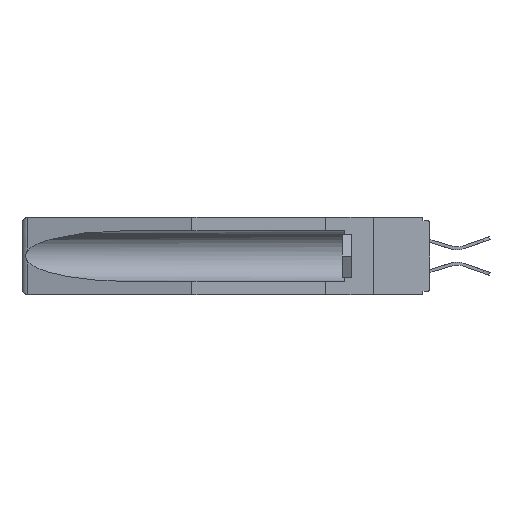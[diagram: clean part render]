
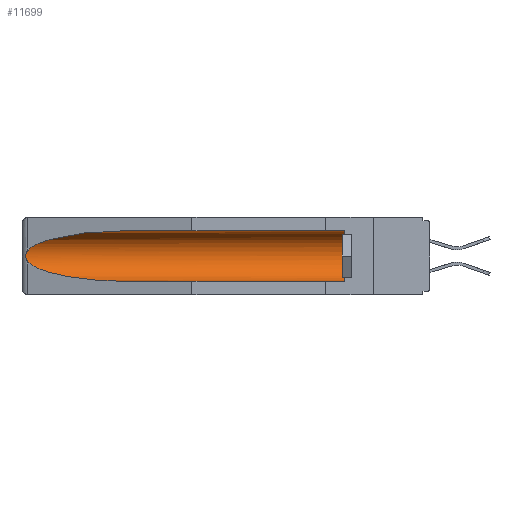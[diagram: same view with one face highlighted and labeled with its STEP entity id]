
A CAD part, left-side view. The second image highlights one B-rep face of the part: STEP entity #11699.
In plain terms, the highlighted cylindrical face has radius 2.857 mm (diameter 5.715 mm), a partial arc.
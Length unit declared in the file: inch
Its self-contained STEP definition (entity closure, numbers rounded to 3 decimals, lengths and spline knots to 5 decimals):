
#415 = VECTOR ( 'NONE', #14873, 39.37008 ) ;
#1009 = EDGE_LOOP ( 'NONE', ( #5394, #13830, #5925, #6684, #20605, #19363 ) ) ;
#1041 = FACE_OUTER_BOUND ( 'NONE', #1009, .T. ) ;
#1133 = EDGE_CURVE ( 'NONE', #16510, #6297, #2123, .T. ) ;
#1208 = B_SPLINE_CURVE_WITH_KNOTS ( 'NONE', 3,
 ( #4345, #9193, #5957, #7654, #20341, #10813, #12405, #2798, #13991, #10535 ),
 .UNSPECIFIED., .F., .F.,
 ( 4, 2, 2, 2, 4 ),
 ( 0., 0.00029, 0.00058, 0.00087, 0.00117 ),
 .UNSPECIFIED. ) ;
#1260 = CIRCLE ( 'NONE', #14836, 0.1125 ) ;
#2104 = CARTESIAN_POINT ( 'NONE',  ( 0.155, 0.126, -0.059 ) ) ;
#2123 =( BOUNDED_CURVE ( )  B_SPLINE_CURVE ( 3, ( #16134, #20662, #11133, #6352 ),
 .UNSPECIFIED., .F., .F. ) 
 B_SPLINE_CURVE_WITH_KNOTS ( ( 4, 4 ),
 ( 0.1948, 1.5708 ),
 .UNSPECIFIED. ) 
 CURVE ( )  GEOMETRIC_REPRESENTATION_ITEM ( )  RATIONAL_B_SPLINE_CURVE ( ( 1., 0.848, 0.848, 1. ) ) 
 REPRESENTATION_ITEM ( '' )  );
#2798 = CARTESIAN_POINT ( 'NONE',  ( 0.26655, 1.53094, -0.18657 ) ) ;
#2909 = DIRECTION ( 'NONE',  ( 0., 1., 0. ) ) ;
#3567 = CARTESIAN_POINT ( 'NONE',  ( 0.155, 0.126, -0.284 ) ) ;
#3704 = CARTESIAN_POINT ( 'NONE',  ( 0.155, -0.30754, -0.059 ) ) ;
#3918 = VERTEX_POINT ( 'NONE', #3567 ) ;
#3929 = LINE ( 'NONE', #3704, #415 ) ;
#4345 = CARTESIAN_POINT ( 'NONE',  ( 0.26537, 1.52718, -0.14972 ) ) ;
#5394 = ORIENTED_EDGE ( 'NONE', *, *, #11500, .T. ) ;
#5925 = ORIENTED_EDGE ( 'NONE', *, *, #1133, .T. ) ;
#5957 = CARTESIAN_POINT ( 'NONE',  ( 0.26654, 1.53092, -0.15636 ) ) ;
#6297 = VERTEX_POINT ( 'NONE', #13156 ) ;
#6352 = CARTESIAN_POINT ( 'NONE',  ( 0.155, 1.07973, -0.284 ) ) ;
#6468 = EDGE_CURVE ( 'NONE', #10651, #13782, #3929, .T. ) ;
#6552 = VECTOR ( 'NONE', #2909, 39.37008 ) ;
#6684 = ORIENTED_EDGE ( 'NONE', *, *, #9178, .F. ) ;
#6819 = CARTESIAN_POINT ( 'NONE',  ( 0.21114, 1.30732, -0.059 ) ) ;
#7586 = CARTESIAN_POINT ( 'NONE',  ( 0.155, 0.126, -0.1715 ) ) ;
#7654 = CARTESIAN_POINT ( 'NONE',  ( 0.2673, 1.5327, -0.16383 ) ) ;
#8056 = CYLINDRICAL_SURFACE ( 'NONE', #12707, 0.1125 ) ;
#8596 = DIRECTION ( 'NONE',  ( 0., 1., 0. ) ) ;
#9178 = EDGE_CURVE ( 'NONE', #3918, #6297, #18513, .T. ) ;
#9193 = CARTESIAN_POINT ( 'NONE',  ( 0.26597, 1.52961, -0.15275 ) ) ;
#9408 = CARTESIAN_POINT ( 'NONE',  ( 0.26537, 1.52718, -0.14972 ) ) ;
#9624 = EDGE_CURVE ( 'NONE', #3918, #10651, #1260, .T. ) ;
#9978 = CARTESIAN_POINT ( 'NONE',  ( 0.26537, 1.52718, -0.14972 ) ) ;
#10113 = VERTEX_POINT ( 'NONE', #9408 ) ;
#10214 =( BOUNDED_CURVE ( )  B_SPLINE_CURVE ( 3, ( #19652, #6819, #19514, #9978 ),
 .UNSPECIFIED., .F., .F. ) 
 B_SPLINE_CURVE_WITH_KNOTS ( ( 4, 4 ),
 ( 4.71239, 6.08839 ),
 .UNSPECIFIED. ) 
 CURVE ( )  GEOMETRIC_REPRESENTATION_ITEM ( )  RATIONAL_B_SPLINE_CURVE ( ( 1., 0.848, 0.848, 1. ) ) 
 REPRESENTATION_ITEM ( '' )  );
#10535 = CARTESIAN_POINT ( 'NONE',  ( 0.26537, 1.52718, -0.19328 ) ) ;
#10651 = VERTEX_POINT ( 'NONE', #2104 ) ;
#10813 = CARTESIAN_POINT ( 'NONE',  ( 0.2675, 1.53308, -0.17534 ) ) ;
#11019 = DIRECTION ( 'NONE',  ( 0., 0., 1. ) ) ;
#11133 = CARTESIAN_POINT ( 'NONE',  ( 0.21114, 1.30732, -0.284 ) ) ;
#11500 = EDGE_CURVE ( 'NONE', #13782, #10113, #10214, .T. ) ;
#11699 = ADVANCED_FACE ( 'NONE', ( #1041 ), #8056, .F. ) ;
#12405 = CARTESIAN_POINT ( 'NONE',  ( 0.2673, 1.53269, -0.17917 ) ) ;
#12707 = AXIS2_PLACEMENT_3D ( 'NONE', #18103, #8596, #15050 ) ;
#13156 = CARTESIAN_POINT ( 'NONE',  ( 0.155, 1.07973, -0.284 ) ) ;
#13782 = VERTEX_POINT ( 'NONE', #18788 ) ;
#13830 = ORIENTED_EDGE ( 'NONE', *, *, #19851, .T. ) ;
#13991 = CARTESIAN_POINT ( 'NONE',  ( 0.26597, 1.5296, -0.19026 ) ) ;
#14836 = AXIS2_PLACEMENT_3D ( 'NONE', #7586, #18938, #11019 ) ;
#14873 = DIRECTION ( 'NONE',  ( 0., 1., 0. ) ) ;
#15050 = DIRECTION ( 'NONE',  ( 0., 0., 1. ) ) ;
#15944 = CARTESIAN_POINT ( 'NONE',  ( 0.26537, 1.52718, -0.19328 ) ) ;
#16134 = CARTESIAN_POINT ( 'NONE',  ( 0.26537, 1.52718, -0.19328 ) ) ;
#16510 = VERTEX_POINT ( 'NONE', #15944 ) ;
#18103 = CARTESIAN_POINT ( 'NONE',  ( 0.155, -0.30754, -0.1715 ) ) ;
#18513 = LINE ( 'NONE', #20374, #6552 ) ;
#18788 = CARTESIAN_POINT ( 'NONE',  ( 0.155, 1.07973, -0.059 ) ) ;
#18938 = DIRECTION ( 'NONE',  ( 0., -1., 0. ) ) ;
#19363 = ORIENTED_EDGE ( 'NONE', *, *, #6468, .T. ) ;
#19514 = CARTESIAN_POINT ( 'NONE',  ( 0.25451, 1.48313, -0.09465 ) ) ;
#19652 = CARTESIAN_POINT ( 'NONE',  ( 0.155, 1.07973, -0.059 ) ) ;
#19851 = EDGE_CURVE ( 'NONE', #10113, #16510, #1208, .T. ) ;
#20341 = CARTESIAN_POINT ( 'NONE',  ( 0.2675, 1.53308, -0.16763 ) ) ;
#20374 = CARTESIAN_POINT ( 'NONE',  ( 0.155, -0.30754, -0.284 ) ) ;
#20605 = ORIENTED_EDGE ( 'NONE', *, *, #9624, .T. ) ;
#20662 = CARTESIAN_POINT ( 'NONE',  ( 0.25451, 1.48313, -0.24835 ) ) ;
